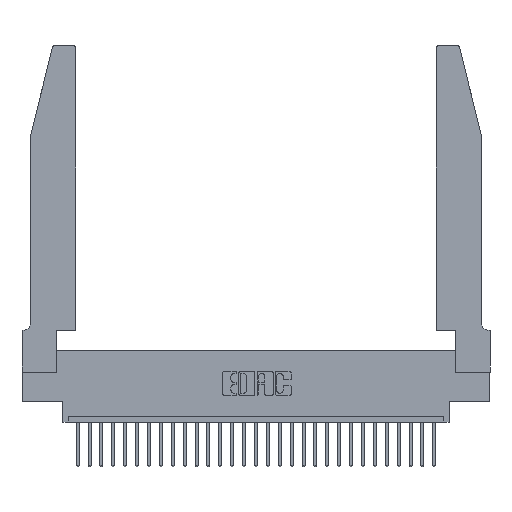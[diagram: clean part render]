
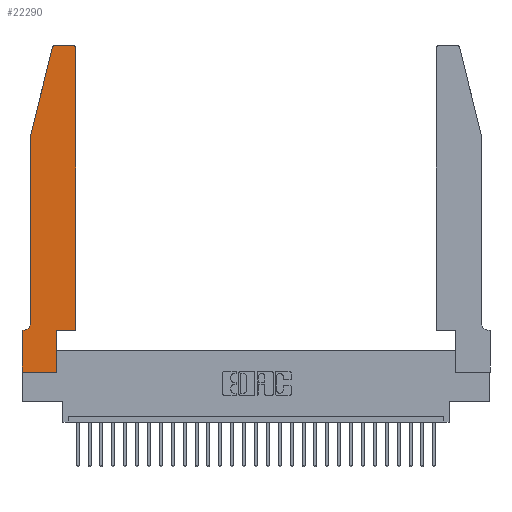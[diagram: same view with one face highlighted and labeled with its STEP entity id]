
A CAD part, top view. The second image highlights one B-rep face of the part: STEP entity #22290.
In plain terms, the highlighted planar face has unit normal (0, 0, 1).
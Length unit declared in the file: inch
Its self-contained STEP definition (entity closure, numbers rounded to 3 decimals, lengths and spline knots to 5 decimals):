
#7 = DIRECTION ( 'NONE',  ( 0., 0., 1. ) ) ;
#84 = VECTOR ( 'NONE', #8602, 39.37008 ) ;
#86 = CARTESIAN_POINT ( 'NONE',  ( 0.2865, 0.35, 0.37 ) ) ;
#184 = DIRECTION ( 'NONE',  ( 0., 0., 1. ) ) ;
#638 = ORIENTED_EDGE ( 'NONE', *, *, #6521, .T. ) ;
#1989 = LINE ( 'NONE', #19525, #25671 ) ;
#2129 = DIRECTION ( 'NONE',  ( 1., 0., 0. ) ) ;
#2509 = CARTESIAN_POINT ( 'NONE',  ( 0., 0., 0.37 ) ) ;
#2606 = AXIS2_PLACEMENT_3D ( 'NONE', #27510, #7, #2129 ) ;
#2674 = CIRCLE ( 'NONE', #14207, 0.07 ) ;
#4030 = DIRECTION ( 'NONE',  ( 0., 0., 1. ) ) ;
#4037 = EDGE_CURVE ( 'NONE', #7422, #12857, #15356, .T. ) ;
#4317 = ORIENTED_EDGE ( 'NONE', *, *, #5389, .T. ) ;
#4360 = PLANE ( 'NONE',  #24663 ) ;
#4640 = CARTESIAN_POINT ( 'NONE',  ( 0.4205, 2.72, 0.37 ) ) ;
#4855 = CARTESIAN_POINT ( 'NONE',  ( 0.2605, 2.75, 0.37 ) ) ;
#4931 = LINE ( 'NONE', #19654, #21806 ) ;
#5389 = EDGE_CURVE ( 'NONE', #22467, #17312, #1989, .T. ) ;
#5409 = ORIENTED_EDGE ( 'NONE', *, *, #23732, .T. ) ;
#5614 = EDGE_CURVE ( 'NONE', #13100, #19836, #9178, .T. ) ;
#5789 = DIRECTION ( 'NONE',  ( -1., 0., 0. ) ) ;
#5845 = CARTESIAN_POINT ( 'NONE',  ( 0.0755, 2., 0.37 ) ) ;
#6258 = DIRECTION ( 'NONE',  ( 1., 0., 0. ) ) ;
#6521 = EDGE_CURVE ( 'NONE', #7132, #7346, #6944, .T. ) ;
#6670 = VECTOR ( 'NONE', #9414, 39.37008 ) ;
#6944 = LINE ( 'NONE', #13312, #84 ) ;
#7132 = VERTEX_POINT ( 'NONE', #18542 ) ;
#7140 = VERTEX_POINT ( 'NONE', #18346 ) ;
#7346 = VERTEX_POINT ( 'NONE', #5845 ) ;
#7422 = VERTEX_POINT ( 'NONE', #14154 ) ;
#8602 = DIRECTION ( 'NONE',  ( -0.239, -0.971, 0. ) ) ;
#9002 = ORIENTED_EDGE ( 'NONE', *, *, #27992, .T. ) ;
#9178 = LINE ( 'NONE', #4855, #6670 ) ;
#9346 = DIRECTION ( 'NONE',  ( -1., 0., 0. ) ) ;
#9414 = DIRECTION ( 'NONE',  ( -1., 0., 0. ) ) ;
#9855 = VERTEX_POINT ( 'NONE', #22132 ) ;
#10368 = ORIENTED_EDGE ( 'NONE', *, *, #27425, .T. ) ;
#10716 = VECTOR ( 'NONE', #15443, 39.37008 ) ;
#10882 = CIRCLE ( 'NONE', #2606, 0.03 ) ;
#11011 = LINE ( 'NONE', #2509, #19958 ) ;
#11060 = CARTESIAN_POINT ( 'NONE',  ( 0., 0.35, 0.37 ) ) ;
#11755 = CARTESIAN_POINT ( 'NONE',  ( 0.0055, 0.42, 0.37 ) ) ;
#12091 = CARTESIAN_POINT ( 'NONE',  ( 0.4505, 0.35, 0.37 ) ) ;
#12159 = CIRCLE ( 'NONE', #13531, 0.03 ) ;
#12857 = VERTEX_POINT ( 'NONE', #19628 ) ;
#13100 = VERTEX_POINT ( 'NONE', #17094 ) ;
#13312 = CARTESIAN_POINT ( 'NONE',  ( 0.0755, 2., 0.37 ) ) ;
#13375 = VECTOR ( 'NONE', #16940, 39.37008 ) ;
#13531 = AXIS2_PLACEMENT_3D ( 'NONE', #4640, #184, #16261 ) ;
#13590 = FACE_OUTER_BOUND ( 'NONE', #23811, .T. ) ;
#14040 = DIRECTION ( 'NONE',  ( 1., 0., 0. ) ) ;
#14154 = CARTESIAN_POINT ( 'NONE',  ( 0.2865, 0.35, 0.37 ) ) ;
#14207 = AXIS2_PLACEMENT_3D ( 'NONE', #11755, #25177, #9346 ) ;
#14305 = ORIENTED_EDGE ( 'NONE', *, *, #4037, .T. ) ;
#15356 = LINE ( 'NONE', #17742, #10716 ) ;
#15443 = DIRECTION ( 'NONE',  ( 1., 0., 0. ) ) ;
#15572 = EDGE_CURVE ( 'NONE', #17312, #22230, #11011, .T. ) ;
#16261 = DIRECTION ( 'NONE',  ( 1., 0., 0. ) ) ;
#16397 = ORIENTED_EDGE ( 'NONE', *, *, #24195, .T. ) ;
#16437 = DIRECTION ( 'NONE',  ( 0., -1., 0. ) ) ;
#16940 = DIRECTION ( 'NONE',  ( 0., 1., 0. ) ) ;
#17094 = CARTESIAN_POINT ( 'NONE',  ( 0.4205, 2.75, 0.37 ) ) ;
#17312 = VERTEX_POINT ( 'NONE', #11060 ) ;
#17385 = EDGE_CURVE ( 'NONE', #7140, #22467, #2674, .T. ) ;
#17527 = LINE ( 'NONE', #12091, #25098 ) ;
#17565 = ORIENTED_EDGE ( 'NONE', *, *, #15572, .T. ) ;
#17708 = ORIENTED_EDGE ( 'NONE', *, *, #27395, .T. ) ;
#17742 = CARTESIAN_POINT ( 'NONE',  ( 0.4505, 0.35, 0.37 ) ) ;
#18346 = CARTESIAN_POINT ( 'NONE',  ( 0.0755, 0.42, 0.37 ) ) ;
#18542 = CARTESIAN_POINT ( 'NONE',  ( 0.25487, 2.72718, 0.37 ) ) ;
#18875 = CARTESIAN_POINT ( 'NONE',  ( 0., 0.35, 0.37 ) ) ;
#19525 = CARTESIAN_POINT ( 'NONE',  ( 0.0755, 0.35, 0.37 ) ) ;
#19628 = CARTESIAN_POINT ( 'NONE',  ( 0.4505, 0.35, 0.37 ) ) ;
#19654 = CARTESIAN_POINT ( 'NONE',  ( 0.0755, 2., 0.37 ) ) ;
#19836 = VERTEX_POINT ( 'NONE', #25818 ) ;
#19958 = VECTOR ( 'NONE', #16437, 39.37008 ) ;
#20491 = CARTESIAN_POINT ( 'NONE',  ( 0., 0., 0.37 ) ) ;
#20877 = LINE ( 'NONE', #20491, #28057 ) ;
#21806 = VECTOR ( 'NONE', #26599, 39.37008 ) ;
#22132 = CARTESIAN_POINT ( 'NONE',  ( 0.4505, 2.72, 0.37 ) ) ;
#22230 = VERTEX_POINT ( 'NONE', #24331 ) ;
#22290 = ADVANCED_FACE ( 'NONE', ( #13590 ), #4360, .T. ) ;
#22331 = LINE ( 'NONE', #86, #13375 ) ;
#22467 = VERTEX_POINT ( 'NONE', #24786 ) ;
#22503 = VERTEX_POINT ( 'NONE', #26804 ) ;
#23333 = ORIENTED_EDGE ( 'NONE', *, *, #24543, .T. ) ;
#23698 = ORIENTED_EDGE ( 'NONE', *, *, #17385, .T. ) ;
#23732 = EDGE_CURVE ( 'NONE', #12857, #9855, #17527, .T. ) ;
#23811 = EDGE_LOOP ( 'NONE', ( #29145, #17708, #638, #23333, #23698, #4317, #17565, #9002, #10368, #14305, #5409, #16397 ) ) ;
#24195 = EDGE_CURVE ( 'NONE', #9855, #13100, #12159, .T. ) ;
#24331 = CARTESIAN_POINT ( 'NONE',  ( 0., 0., 0.37 ) ) ;
#24543 = EDGE_CURVE ( 'NONE', #7346, #7140, #4931, .T. ) ;
#24663 = AXIS2_PLACEMENT_3D ( 'NONE', #18875, #4030, #6258 ) ;
#24786 = CARTESIAN_POINT ( 'NONE',  ( 0.0055, 0.35, 0.37 ) ) ;
#25098 = VECTOR ( 'NONE', #25426, 39.37008 ) ;
#25177 = DIRECTION ( 'NONE',  ( 0., 0., -1. ) ) ;
#25426 = DIRECTION ( 'NONE',  ( 0., 1., 0. ) ) ;
#25671 = VECTOR ( 'NONE', #5789, 39.37008 ) ;
#25818 = CARTESIAN_POINT ( 'NONE',  ( 0.284, 2.75, 0.37 ) ) ;
#26599 = DIRECTION ( 'NONE',  ( 0., -1., 0. ) ) ;
#26804 = CARTESIAN_POINT ( 'NONE',  ( 0.2865, 0., 0.37 ) ) ;
#27395 = EDGE_CURVE ( 'NONE', #19836, #7132, #10882, .T. ) ;
#27425 = EDGE_CURVE ( 'NONE', #22503, #7422, #22331, .T. ) ;
#27510 = CARTESIAN_POINT ( 'NONE',  ( 0.284, 2.72, 0.37 ) ) ;
#27992 = EDGE_CURVE ( 'NONE', #22230, #22503, #20877, .T. ) ;
#28057 = VECTOR ( 'NONE', #14040, 39.37008 ) ;
#29145 = ORIENTED_EDGE ( 'NONE', *, *, #5614, .T. ) ;
